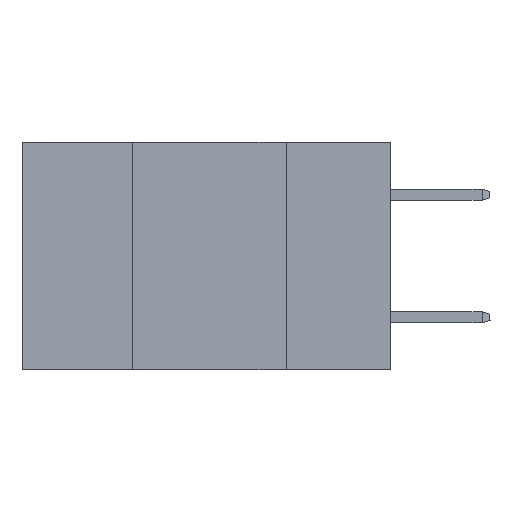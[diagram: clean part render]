
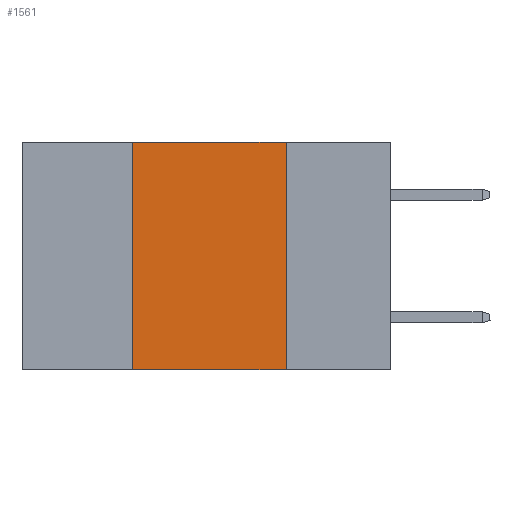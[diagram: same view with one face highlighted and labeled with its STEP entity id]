
A CAD part, left-side view. The second image highlights one B-rep face of the part: STEP entity #1561.
In plain terms, the highlighted planar face has unit normal (-1, 0, 0).
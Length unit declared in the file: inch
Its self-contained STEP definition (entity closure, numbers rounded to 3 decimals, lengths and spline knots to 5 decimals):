
#119 = ORIENTED_EDGE ( 'NONE', *, *, #12224, .F. ) ;
#576 = LINE ( 'NONE', #12017, #5356 ) ;
#785 = DIRECTION ( 'NONE',  ( 1., 0., 0. ) ) ;
#1358 = LINE ( 'NONE', #8907, #4948 ) ;
#1417 = VERTEX_POINT ( 'NONE', #10721 ) ;
#1561 = ADVANCED_FACE ( 'NONE', ( #4246 ), #9341, .F. ) ;
#1691 = CARTESIAN_POINT ( 'NONE',  ( 0., 0.17, 0. ) ) ;
#1712 = EDGE_CURVE ( 'NONE', #7819, #5147, #6913, .T. ) ;
#1762 = DIRECTION ( 'NONE',  ( 0., 0., -1. ) ) ;
#2491 = VERTEX_POINT ( 'NONE', #3828 ) ;
#2718 = DIRECTION ( 'NONE',  ( 0., 0., -1. ) ) ;
#2831 = EDGE_CURVE ( 'NONE', #7819, #2491, #1358, .T. ) ;
#3436 = ORIENTED_EDGE ( 'NONE', *, *, #2831, .F. ) ;
#3462 = VECTOR ( 'NONE', #9572, 39.37008 ) ;
#3557 = EDGE_CURVE ( 'NONE', #2491, #1417, #576, .T. ) ;
#3685 = CARTESIAN_POINT ( 'NONE',  ( 0., 0.17, -0.37 ) ) ;
#3828 = CARTESIAN_POINT ( 'NONE',  ( 0., 0.42, 0. ) ) ;
#3930 = CARTESIAN_POINT ( 'NONE',  ( 0., 0.6, -0.37 ) ) ;
#4246 = FACE_OUTER_BOUND ( 'NONE', #7844, .T. ) ;
#4948 = VECTOR ( 'NONE', #11795, 39.37008 ) ;
#4999 = ORIENTED_EDGE ( 'NONE', *, *, #3557, .F. ) ;
#5147 = VERTEX_POINT ( 'NONE', #3685 ) ;
#5356 = VECTOR ( 'NONE', #6291, 39.37008 ) ;
#6291 = DIRECTION ( 'NONE',  ( 0., -1., 0. ) ) ;
#6494 = VECTOR ( 'NONE', #2718, 39.37008 ) ;
#6789 = LINE ( 'NONE', #1691, #6494 ) ;
#6913 = LINE ( 'NONE', #3930, #3462 ) ;
#7819 = VERTEX_POINT ( 'NONE', #9563 ) ;
#7844 = EDGE_LOOP ( 'NONE', ( #119, #4999, #3436, #9967 ) ) ;
#8907 = CARTESIAN_POINT ( 'NONE',  ( 0., 0.42, 0. ) ) ;
#9341 = PLANE ( 'NONE',  #9893 ) ;
#9563 = CARTESIAN_POINT ( 'NONE',  ( 0., 0.42, -0.37 ) ) ;
#9572 = DIRECTION ( 'NONE',  ( 0., -1., 0. ) ) ;
#9893 = AXIS2_PLACEMENT_3D ( 'NONE', #10285, #785, #1762 ) ;
#9967 = ORIENTED_EDGE ( 'NONE', *, *, #1712, .T. ) ;
#10285 = CARTESIAN_POINT ( 'NONE',  ( 0., 0.6, 0. ) ) ;
#10721 = CARTESIAN_POINT ( 'NONE',  ( 0., 0.17, 0. ) ) ;
#11795 = DIRECTION ( 'NONE',  ( 0., 0., 1. ) ) ;
#12017 = CARTESIAN_POINT ( 'NONE',  ( 0., 0.6, 0. ) ) ;
#12224 = EDGE_CURVE ( 'NONE', #1417, #5147, #6789, .T. ) ;
